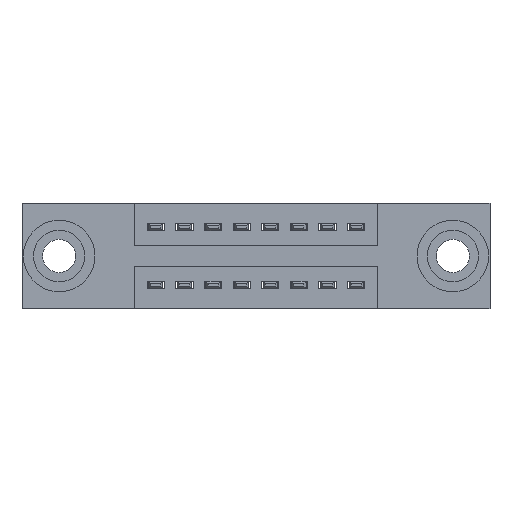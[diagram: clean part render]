
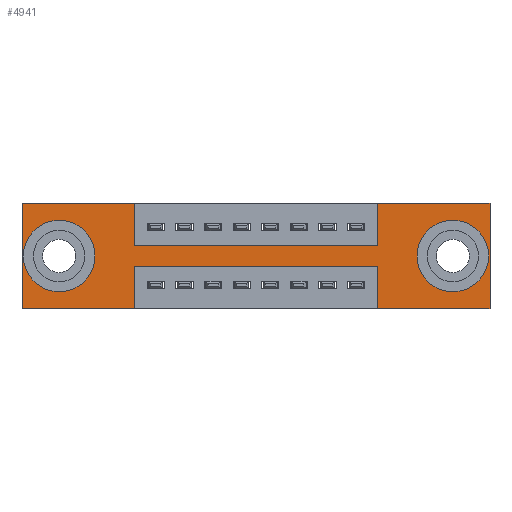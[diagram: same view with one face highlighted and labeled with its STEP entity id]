
A CAD part, front view. The second image highlights one B-rep face of the part: STEP entity #4941.
In plain terms, the highlighted planar face has unit normal (0, -1, 0).
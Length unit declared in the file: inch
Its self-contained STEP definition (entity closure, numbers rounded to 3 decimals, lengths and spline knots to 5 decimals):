
#85 = EDGE_CURVE ( 'NONE', #3269, #3825, #10048, .T. ) ;
#153 = VERTEX_POINT ( 'NONE', #6899 ) ;
#204 = CARTESIAN_POINT ( 'NONE',  ( 0., 0., -0.37 ) ) ;
#372 = CARTESIAN_POINT ( 'NONE',  ( 1.505, 0., -0.263 ) ) ;
#626 = DIRECTION ( 'NONE',  ( 0., 0., -1. ) ) ;
#721 = VECTOR ( 'NONE', #4971, 39.37008 ) ;
#919 = DIRECTION ( 'NONE',  ( 0., 1., 0. ) ) ;
#979 = LINE ( 'NONE', #2278, #9369 ) ;
#1009 = ORIENTED_EDGE ( 'NONE', *, *, #8880, .F. ) ;
#1298 = ORIENTED_EDGE ( 'NONE', *, *, #9342, .T. ) ;
#1320 = DIRECTION ( 'NONE',  ( 0., 0., -1. ) ) ;
#1322 = EDGE_LOOP ( 'NONE', ( #1298, #1681 ) ) ;
#1391 = CARTESIAN_POINT ( 'NONE',  ( 1.635, 0., 0. ) ) ;
#1394 = ORIENTED_EDGE ( 'NONE', *, *, #4988, .F. ) ;
#1607 = FACE_BOUND ( 'NONE', #5388, .T. ) ;
#1625 = VERTEX_POINT ( 'NONE', #9793 ) ;
#1681 = ORIENTED_EDGE ( 'NONE', *, *, #3059, .T. ) ;
#1833 = ORIENTED_EDGE ( 'NONE', *, *, #10677, .T. ) ;
#1936 = CARTESIAN_POINT ( 'NONE',  ( 0.3925, 0., -0.15 ) ) ;
#1955 = ORIENTED_EDGE ( 'NONE', *, *, #3653, .F. ) ;
#2080 = CIRCLE ( 'NONE', #7960, 0.078 ) ;
#2204 = CARTESIAN_POINT ( 'NONE',  ( 0., 0., 0. ) ) ;
#2278 = CARTESIAN_POINT ( 'NONE',  ( 0., 0., 0. ) ) ;
#2432 = EDGE_CURVE ( 'NONE', #3904, #6644, #4242, .T. ) ;
#2474 = LINE ( 'NONE', #10298, #3123 ) ;
#2511 = VERTEX_POINT ( 'NONE', #10878 ) ;
#2521 = CARTESIAN_POINT ( 'NONE',  ( 0., 0., -0.37 ) ) ;
#2545 = ORIENTED_EDGE ( 'NONE', *, *, #2432, .T. ) ;
#2572 = ORIENTED_EDGE ( 'NONE', *, *, #8621, .F. ) ;
#2695 = EDGE_CURVE ( 'NONE', #7666, #2511, #3827, .T. ) ;
#2836 = VECTOR ( 'NONE', #3167, 39.37008 ) ;
#2868 = ORIENTED_EDGE ( 'NONE', *, *, #2695, .F. ) ;
#3040 = LINE ( 'NONE', #9340, #721 ) ;
#3059 = EDGE_CURVE ( 'NONE', #11096, #153, #9613, .T. ) ;
#3096 = VERTEX_POINT ( 'NONE', #6585 ) ;
#3114 = CARTESIAN_POINT ( 'NONE',  ( 0.13, 0., -0.185 ) ) ;
#3123 = VECTOR ( 'NONE', #6040, 39.37008 ) ;
#3130 = CARTESIAN_POINT ( 'NONE',  ( 0.3925, 0., -0.22 ) ) ;
#3167 = DIRECTION ( 'NONE',  ( 0., 0., 1. ) ) ;
#3258 = CARTESIAN_POINT ( 'NONE',  ( 1.505, 0., -0.107 ) ) ;
#3269 = VERTEX_POINT ( 'NONE', #8135 ) ;
#3548 = DIRECTION ( 'NONE',  ( 0., 0., 1. ) ) ;
#3579 = DIRECTION ( 'NONE',  ( 0., 0., -1. ) ) ;
#3653 = EDGE_CURVE ( 'NONE', #8444, #8614, #6024, .T. ) ;
#3665 = DIRECTION ( 'NONE',  ( 1., 0., 0. ) ) ;
#3825 = VERTEX_POINT ( 'NONE', #6655 ) ;
#3827 = LINE ( 'NONE', #1391, #11103 ) ;
#3903 = VERTEX_POINT ( 'NONE', #5168 ) ;
#3904 = VERTEX_POINT ( 'NONE', #3258 ) ;
#4242 = CIRCLE ( 'NONE', #7400, 0.078 ) ;
#4488 = EDGE_CURVE ( 'NONE', #3096, #8444, #6240, .T. ) ;
#4562 = ORIENTED_EDGE ( 'NONE', *, *, #10965, .F. ) ;
#4653 = CARTESIAN_POINT ( 'NONE',  ( 1.635, 0., 0. ) ) ;
#4718 = AXIS2_PLACEMENT_3D ( 'NONE', #8004, #6311, #3579 ) ;
#4941 = ADVANCED_FACE ( 'NONE', ( #1607, #7631, #5291 ), #5250, .T. ) ;
#4971 = DIRECTION ( 'NONE',  ( 0., 0., -1. ) ) ;
#4988 = EDGE_CURVE ( 'NONE', #9898, #1625, #11048, .T. ) ;
#5034 = LINE ( 'NONE', #10086, #9596 ) ;
#5125 = EDGE_CURVE ( 'NONE', #3903, #3269, #10623, .T. ) ;
#5168 = CARTESIAN_POINT ( 'NONE',  ( 0.3925, 0., -0.15 ) ) ;
#5250 = PLANE ( 'NONE',  #5287 ) ;
#5287 = AXIS2_PLACEMENT_3D ( 'NONE', #204, #10734, #1320 ) ;
#5291 = FACE_OUTER_BOUND ( 'NONE', #9761, .T. ) ;
#5349 = EDGE_CURVE ( 'NONE', #8614, #3903, #5689, .T. ) ;
#5388 = EDGE_LOOP ( 'NONE', ( #2545, #1833 ) ) ;
#5672 = ORIENTED_EDGE ( 'NONE', *, *, #5125, .F. ) ;
#5689 = LINE ( 'NONE', #8883, #7763 ) ;
#5901 = CARTESIAN_POINT ( 'NONE',  ( 0.3925, 0., 0. ) ) ;
#5932 = CARTESIAN_POINT ( 'NONE',  ( 0.3925, 0., -0.37 ) ) ;
#6024 = LINE ( 'NONE', #7356, #9733 ) ;
#6040 = DIRECTION ( 'NONE',  ( -1., 0., 0. ) ) ;
#6134 = CIRCLE ( 'NONE', #4718, 0.078 ) ;
#6240 = LINE ( 'NONE', #2204, #2836 ) ;
#6296 = DIRECTION ( 'NONE',  ( 0., 0., -1. ) ) ;
#6311 = DIRECTION ( 'NONE',  ( 0., 1., 0. ) ) ;
#6319 = CARTESIAN_POINT ( 'NONE',  ( 1.2425, 0., -0.37 ) ) ;
#6459 = DIRECTION ( 'NONE',  ( 1., 0., 0. ) ) ;
#6574 = ORIENTED_EDGE ( 'NONE', *, *, #4488, .F. ) ;
#6582 = DIRECTION ( 'NONE',  ( 0., 0., 1. ) ) ;
#6584 = DIRECTION ( 'NONE',  ( 0., 0., 1. ) ) ;
#6585 = CARTESIAN_POINT ( 'NONE',  ( 0., 0., -0.37 ) ) ;
#6644 = VERTEX_POINT ( 'NONE', #372 ) ;
#6655 = CARTESIAN_POINT ( 'NONE',  ( 1.2425, 0., 0. ) ) ;
#6899 = CARTESIAN_POINT ( 'NONE',  ( 0.13, 0., -0.107 ) ) ;
#7333 = VECTOR ( 'NONE', #3665, 39.37008 ) ;
#7356 = CARTESIAN_POINT ( 'NONE',  ( 0., 0., 0. ) ) ;
#7400 = AXIS2_PLACEMENT_3D ( 'NONE', #9846, #9994, #9095 ) ;
#7631 = FACE_BOUND ( 'NONE', #1322, .T. ) ;
#7666 = VERTEX_POINT ( 'NONE', #4653 ) ;
#7763 = VECTOR ( 'NONE', #6296, 39.37008 ) ;
#7960 = AXIS2_PLACEMENT_3D ( 'NONE', #3114, #9279, #6584 ) ;
#8001 = VERTEX_POINT ( 'NONE', #5932 ) ;
#8004 = CARTESIAN_POINT ( 'NONE',  ( 1.505, 0., -0.185 ) ) ;
#8095 = CARTESIAN_POINT ( 'NONE',  ( 1.2425, 0., -0.37 ) ) ;
#8135 = CARTESIAN_POINT ( 'NONE',  ( 1.2425, 0., -0.15 ) ) ;
#8177 = DIRECTION ( 'NONE',  ( 0., 0., 1. ) ) ;
#8444 = VERTEX_POINT ( 'NONE', #10244 ) ;
#8494 = VERTEX_POINT ( 'NONE', #3130 ) ;
#8614 = VERTEX_POINT ( 'NONE', #5901 ) ;
#8621 = EDGE_CURVE ( 'NONE', #8494, #8001, #3040, .T. ) ;
#8623 = AXIS2_PLACEMENT_3D ( 'NONE', #9667, #919, #3548 ) ;
#8740 = EDGE_CURVE ( 'NONE', #8001, #3096, #9517, .T. ) ;
#8880 = EDGE_CURVE ( 'NONE', #3825, #7666, #979, .T. ) ;
#8883 = CARTESIAN_POINT ( 'NONE',  ( 0.3925, 0., 0. ) ) ;
#9020 = CARTESIAN_POINT ( 'NONE',  ( 1.2425, 0., 0. ) ) ;
#9095 = DIRECTION ( 'NONE',  ( 0., 0., -1. ) ) ;
#9279 = DIRECTION ( 'NONE',  ( 0., 1., 0. ) ) ;
#9340 = CARTESIAN_POINT ( 'NONE',  ( 0.3925, 0., -0.37 ) ) ;
#9342 = EDGE_CURVE ( 'NONE', #153, #11096, #2080, .T. ) ;
#9369 = VECTOR ( 'NONE', #10179, 39.37008 ) ;
#9517 = LINE ( 'NONE', #2521, #11130 ) ;
#9596 = VECTOR ( 'NONE', #10333, 39.37008 ) ;
#9613 = CIRCLE ( 'NONE', #8623, 0.078 ) ;
#9620 = CARTESIAN_POINT ( 'NONE',  ( 0.13, 0., -0.263 ) ) ;
#9667 = CARTESIAN_POINT ( 'NONE',  ( 0.13, 0., -0.185 ) ) ;
#9733 = VECTOR ( 'NONE', #6459, 39.37008 ) ;
#9761 = EDGE_LOOP ( 'NONE', ( #2572, #9798, #1394, #4562, #2868, #1009, #10525, #5672, #10980, #1955, #6574, #11256 ) ) ;
#9793 = CARTESIAN_POINT ( 'NONE',  ( 1.2425, 0., -0.22 ) ) ;
#9798 = ORIENTED_EDGE ( 'NONE', *, *, #10142, .F. ) ;
#9846 = CARTESIAN_POINT ( 'NONE',  ( 1.505, 0., -0.185 ) ) ;
#9898 = VERTEX_POINT ( 'NONE', #6319 ) ;
#9922 = VECTOR ( 'NONE', #6582, 39.37008 ) ;
#9994 = DIRECTION ( 'NONE',  ( 0., 1., 0. ) ) ;
#10048 = LINE ( 'NONE', #9020, #9922 ) ;
#10086 = CARTESIAN_POINT ( 'NONE',  ( 0., 0., -0.37 ) ) ;
#10142 = EDGE_CURVE ( 'NONE', #1625, #8494, #2474, .T. ) ;
#10179 = DIRECTION ( 'NONE',  ( 1., 0., 0. ) ) ;
#10244 = CARTESIAN_POINT ( 'NONE',  ( 0., 0., 0. ) ) ;
#10298 = CARTESIAN_POINT ( 'NONE',  ( 0.3925, 0., -0.22 ) ) ;
#10333 = DIRECTION ( 'NONE',  ( -1., 0., 0. ) ) ;
#10510 = DIRECTION ( 'NONE',  ( -1., 0., 0. ) ) ;
#10525 = ORIENTED_EDGE ( 'NONE', *, *, #85, .F. ) ;
#10623 = LINE ( 'NONE', #1936, #7333 ) ;
#10634 = VECTOR ( 'NONE', #8177, 39.37008 ) ;
#10677 = EDGE_CURVE ( 'NONE', #6644, #3904, #6134, .T. ) ;
#10734 = DIRECTION ( 'NONE',  ( 0., -1., 0. ) ) ;
#10878 = CARTESIAN_POINT ( 'NONE',  ( 1.635, 0., -0.37 ) ) ;
#10965 = EDGE_CURVE ( 'NONE', #2511, #9898, #5034, .T. ) ;
#10980 = ORIENTED_EDGE ( 'NONE', *, *, #5349, .F. ) ;
#11048 = LINE ( 'NONE', #8095, #10634 ) ;
#11096 = VERTEX_POINT ( 'NONE', #9620 ) ;
#11103 = VECTOR ( 'NONE', #626, 39.37008 ) ;
#11130 = VECTOR ( 'NONE', #10510, 39.37008 ) ;
#11256 = ORIENTED_EDGE ( 'NONE', *, *, #8740, .F. ) ;
